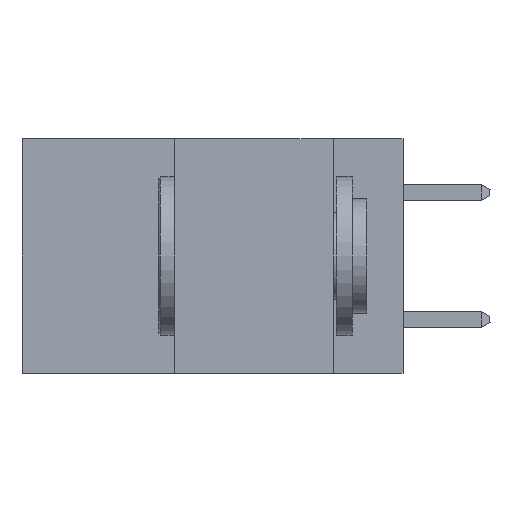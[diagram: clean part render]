
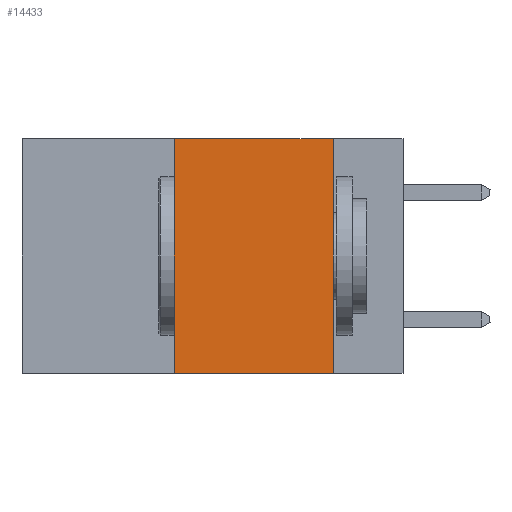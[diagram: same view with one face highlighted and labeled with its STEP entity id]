
A CAD part, left-side view. The second image highlights one B-rep face of the part: STEP entity #14433.
In plain terms, the highlighted planar face has unit normal (-1, 0, 0).
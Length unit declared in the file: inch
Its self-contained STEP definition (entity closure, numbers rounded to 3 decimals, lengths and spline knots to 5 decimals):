
#601 = EDGE_CURVE ( 'NONE', #14639, #19501, #14252, .T. ) ;
#1027 = CARTESIAN_POINT ( 'NONE',  ( 0., 0.6, 0. ) ) ;
#1094 = DIRECTION ( 'NONE',  ( 0., 0., -1. ) ) ;
#1975 = CARTESIAN_POINT ( 'NONE',  ( 0., 0.11, 0. ) ) ;
#2848 = VECTOR ( 'NONE', #5795, 39.37008 ) ;
#4253 = LINE ( 'NONE', #20624, #7802 ) ;
#4455 = EDGE_CURVE ( 'NONE', #5809, #11394, #4253, .T. ) ;
#5131 = EDGE_CURVE ( 'NONE', #14639, #11394, #20903, .T. ) ;
#5189 = VECTOR ( 'NONE', #6567, 39.37008 ) ;
#5795 = DIRECTION ( 'NONE',  ( 0., -1., 0. ) ) ;
#5809 = VERTEX_POINT ( 'NONE', #1975 ) ;
#5902 = CARTESIAN_POINT ( 'NONE',  ( 0., 0.6, -0.37 ) ) ;
#6323 = VECTOR ( 'NONE', #20337, 39.37008 ) ;
#6567 = DIRECTION ( 'NONE',  ( 0., 0., 1. ) ) ;
#6634 = CARTESIAN_POINT ( 'NONE',  ( 0., 0.36, 0. ) ) ;
#7802 = VECTOR ( 'NONE', #20381, 39.37008 ) ;
#8509 = ORIENTED_EDGE ( 'NONE', *, *, #5131, .T. ) ;
#9028 = ORIENTED_EDGE ( 'NONE', *, *, #4455, .F. ) ;
#10447 = AXIS2_PLACEMENT_3D ( 'NONE', #1027, #11498, #1094 ) ;
#11394 = VERTEX_POINT ( 'NONE', #15958 ) ;
#11498 = DIRECTION ( 'NONE',  ( 1., 0., 0. ) ) ;
#11690 = EDGE_LOOP ( 'NONE', ( #9028, #20077, #19324, #8509 ) ) ;
#13465 = EDGE_CURVE ( 'NONE', #19501, #5809, #19805, .T. ) ;
#14252 = LINE ( 'NONE', #6634, #5189 ) ;
#14433 = ADVANCED_FACE ( 'NONE', ( #16616 ), #16490, .F. ) ;
#14639 = VERTEX_POINT ( 'NONE', #21931 ) ;
#15154 = CARTESIAN_POINT ( 'NONE',  ( 0., 0.36, 0. ) ) ;
#15958 = CARTESIAN_POINT ( 'NONE',  ( 0., 0.11, -0.37 ) ) ;
#16490 = PLANE ( 'NONE',  #10447 ) ;
#16616 = FACE_OUTER_BOUND ( 'NONE', #11690, .T. ) ;
#19324 = ORIENTED_EDGE ( 'NONE', *, *, #601, .F. ) ;
#19501 = VERTEX_POINT ( 'NONE', #15154 ) ;
#19805 = LINE ( 'NONE', #20268, #6323 ) ;
#20077 = ORIENTED_EDGE ( 'NONE', *, *, #13465, .F. ) ;
#20268 = CARTESIAN_POINT ( 'NONE',  ( 0., 0.6, 0. ) ) ;
#20337 = DIRECTION ( 'NONE',  ( 0., -1., 0. ) ) ;
#20381 = DIRECTION ( 'NONE',  ( 0., 0., -1. ) ) ;
#20624 = CARTESIAN_POINT ( 'NONE',  ( 0., 0.11, 0. ) ) ;
#20903 = LINE ( 'NONE', #5902, #2848 ) ;
#21931 = CARTESIAN_POINT ( 'NONE',  ( 0., 0.36, -0.37 ) ) ;
